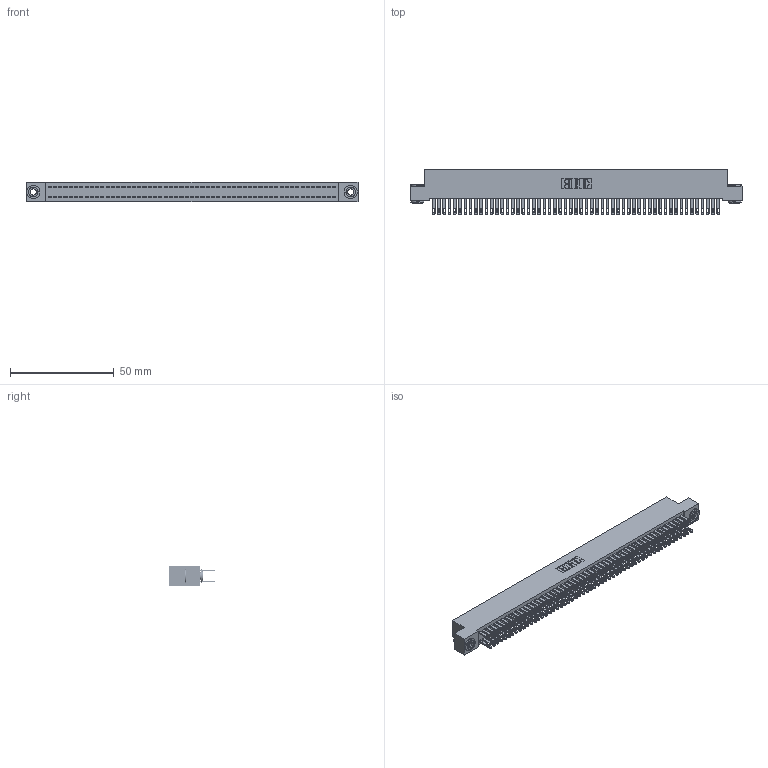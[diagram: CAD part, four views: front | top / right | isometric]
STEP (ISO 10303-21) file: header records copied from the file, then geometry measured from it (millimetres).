
FILE_DESCRIPTION (( 'STEP AP203' ), '1' );
FILE_NAME ('342-110-500-203.STEP', '2018-08-14T11:15:24', ( '' ), ( '' ), 'SwSTEP 2.0', 'SolidWorks 2016', '' );
FILE_SCHEMA (( 'CONFIG_CONTROL_DESIGN' ));
Length unit declared in the file: inch
Products named in the file (4): 342 Part_.156 TH; 345-292-001_345-293-100; 342-250-002_345-250-002-102; 342-110-500-203
Assembly tree (113 placements, depth 2):
  342-110-500-203
    342 Part_.156 TH
    345-292-001_345-293-100  x110
    342-250-002_345-250-002-102  x2
Bounding box: 160.02 x 21.85 x 9.4 mm (x, y, z)
Volume: 14798.3 mm3; surface area: 25675.5 mm2
Topology: 113 solids, 113 shells, 5428 faces, 16545 edges, 11026 vertices
Faces by surface type: plane 3376, cylinder 2044, cone 8
Entity records: 34150 total; most frequent: CARTESIAN_POINT 5617, ORIENTED_EDGE 5546, DIRECTION 4811, EDGE_CURVE 2773, LINE 2617, VECTOR 2617, VERTEX_POINT 1846, AXIS2_PLACEMENT_3D 1097
